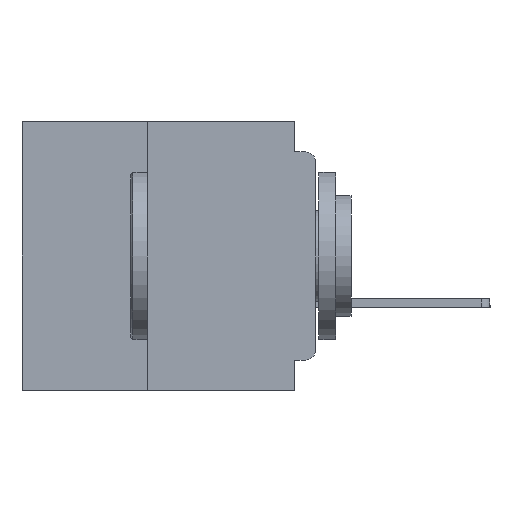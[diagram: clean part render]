
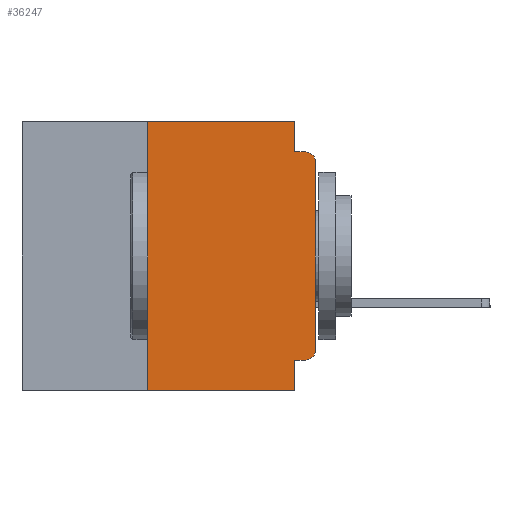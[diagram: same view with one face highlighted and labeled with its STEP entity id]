
A CAD part, left-side view. The second image highlights one B-rep face of the part: STEP entity #36247.
In plain terms, the highlighted planar face has unit normal (-1, 0, 0).
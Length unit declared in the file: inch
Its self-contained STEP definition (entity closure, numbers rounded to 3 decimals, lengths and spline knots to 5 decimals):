
#395 = ORIENTED_EDGE ( 'NONE', *, *, #25275, .F. ) ;
#446 = EDGE_CURVE ( 'NONE', #2039, #25079, #13232, .T. ) ;
#483 = VECTOR ( 'NONE', #23274, 39.37008 ) ;
#754 = AXIS2_PLACEMENT_3D ( 'NONE', #5023, #29631, #8598 ) ;
#2039 = VERTEX_POINT ( 'NONE', #27546 ) ;
#3503 = VECTOR ( 'NONE', #42438, 39.37008 ) ;
#3604 = CIRCLE ( 'NONE', #41711, 0.015 ) ;
#3723 = CARTESIAN_POINT ( 'NONE',  ( 0., 0., -0.06 ) ) ;
#4589 = LINE ( 'NONE', #10989, #3503 ) ;
#5023 = CARTESIAN_POINT ( 'NONE',  ( 0., 0.437, 0. ) ) ;
#5194 = CARTESIAN_POINT ( 'NONE',  ( 0., 0.031, -0.4 ) ) ;
#5878 = CARTESIAN_POINT ( 'NONE',  ( 0., 0.031, -0.4 ) ) ;
#6383 = CARTESIAN_POINT ( 'NONE',  ( 0., 0.031, -0.355 ) ) ;
#6879 = VECTOR ( 'NONE', #44340, 39.37008 ) ;
#7623 = LINE ( 'NONE', #41251, #25225 ) ;
#7993 = AXIS2_PLACEMENT_3D ( 'NONE', #16415, #40830, #19951 ) ;
#8598 = DIRECTION ( 'NONE',  ( 0., 0., -1. ) ) ;
#9558 = ORIENTED_EDGE ( 'NONE', *, *, #15839, .F. ) ;
#9812 = EDGE_LOOP ( 'NONE', ( #27201, #44619, #27132, #28868, #9558, #395, #15084, #21451, #10357, #39577 ) ) ;
#10357 = ORIENTED_EDGE ( 'NONE', *, *, #446, .F. ) ;
#10989 = CARTESIAN_POINT ( 'NONE',  ( 0., 0.25, -0.4 ) ) ;
#11476 = VERTEX_POINT ( 'NONE', #43487 ) ;
#11868 = VECTOR ( 'NONE', #21684, 39.37008 ) ;
#12279 = DIRECTION ( 'NONE',  ( 0., 0., 1. ) ) ;
#12887 = EDGE_CURVE ( 'NONE', #2039, #37448, #28032, .T. ) ;
#13232 = LINE ( 'NONE', #26518, #30829 ) ;
#13358 = VERTEX_POINT ( 'NONE', #26187 ) ;
#15084 = ORIENTED_EDGE ( 'NONE', *, *, #32418, .T. ) ;
#15514 = PLANE ( 'NONE',  #754 ) ;
#15839 = EDGE_CURVE ( 'NONE', #16154, #13358, #7623, .T. ) ;
#16154 = VERTEX_POINT ( 'NONE', #39728 ) ;
#16415 = CARTESIAN_POINT ( 'NONE',  ( 0., 0.015, -0.34 ) ) ;
#16901 = LINE ( 'NONE', #45179, #43590 ) ;
#17373 = DIRECTION ( 'NONE',  ( 0., -1., 0. ) ) ;
#17831 = DIRECTION ( 'NONE',  ( -1., 0., 0. ) ) ;
#18166 = EDGE_CURVE ( 'NONE', #13358, #20723, #30558, .T. ) ;
#18183 = CARTESIAN_POINT ( 'NONE',  ( 0., 0.031, 0. ) ) ;
#18848 = CARTESIAN_POINT ( 'NONE',  ( 0., 0.031, -0.045 ) ) ;
#19744 = CARTESIAN_POINT ( 'NONE',  ( 0., 0.437, -0.4 ) ) ;
#19951 = DIRECTION ( 'NONE',  ( 0., 0., -1. ) ) ;
#20604 = CARTESIAN_POINT ( 'NONE',  ( 0., 0.015, -0.045 ) ) ;
#20723 = VERTEX_POINT ( 'NONE', #18848 ) ;
#21451 = ORIENTED_EDGE ( 'NONE', *, *, #34818, .F. ) ;
#21684 = DIRECTION ( 'NONE',  ( 0., 0., -1. ) ) ;
#22727 = CARTESIAN_POINT ( 'NONE',  ( 0., 0., 0. ) ) ;
#23274 = DIRECTION ( 'NONE',  ( 0., -1., 0. ) ) ;
#24052 = DIRECTION ( 'NONE',  ( 0., -1., 0. ) ) ;
#25079 = VERTEX_POINT ( 'NONE', #6383 ) ;
#25225 = VECTOR ( 'NONE', #24052, 39.37008 ) ;
#25275 = EDGE_CURVE ( 'NONE', #11476, #16154, #4589, .T. ) ;
#26187 = CARTESIAN_POINT ( 'NONE',  ( 0., 0.031, 0. ) ) ;
#26315 = CARTESIAN_POINT ( 'NONE',  ( 0., 0., -0.34 ) ) ;
#26518 = CARTESIAN_POINT ( 'NONE',  ( 0., 0., -0.355 ) ) ;
#27132 = ORIENTED_EDGE ( 'NONE', *, *, #33754, .F. ) ;
#27201 = ORIENTED_EDGE ( 'NONE', *, *, #38030, .T. ) ;
#27368 = DIRECTION ( 'NONE',  ( 0., 1., 0. ) ) ;
#27546 = CARTESIAN_POINT ( 'NONE',  ( 0., 0.015, -0.355 ) ) ;
#28032 = CIRCLE ( 'NONE', #7993, 0.015 ) ;
#28575 = LINE ( 'NONE', #19744, #483 ) ;
#28802 = FACE_OUTER_BOUND ( 'NONE', #9812, .T. ) ;
#28868 = ORIENTED_EDGE ( 'NONE', *, *, #18166, .F. ) ;
#29631 = DIRECTION ( 'NONE',  ( 1., 0., 0. ) ) ;
#30558 = LINE ( 'NONE', #18183, #11868 ) ;
#30829 = VECTOR ( 'NONE', #27368, 39.37008 ) ;
#32418 = EDGE_CURVE ( 'NONE', #11476, #38021, #28575, .T. ) ;
#32707 = VERTEX_POINT ( 'NONE', #3723 ) ;
#33717 = VERTEX_POINT ( 'NONE', #20604 ) ;
#33754 = EDGE_CURVE ( 'NONE', #20723, #33717, #16901, .T. ) ;
#34818 = EDGE_CURVE ( 'NONE', #25079, #38021, #34927, .T. ) ;
#34927 = LINE ( 'NONE', #5878, #6879 ) ;
#36247 = ADVANCED_FACE ( 'NONE', ( #28802 ), #15514, .F. ) ;
#37250 = LINE ( 'NONE', #22727, #45234 ) ;
#37448 = VERTEX_POINT ( 'NONE', #26315 ) ;
#38021 = VERTEX_POINT ( 'NONE', #5194 ) ;
#38030 = EDGE_CURVE ( 'NONE', #37448, #32707, #37250, .T. ) ;
#38776 = CARTESIAN_POINT ( 'NONE',  ( 0., 0.015, -0.06 ) ) ;
#39440 = EDGE_CURVE ( 'NONE', #32707, #33717, #3604, .T. ) ;
#39577 = ORIENTED_EDGE ( 'NONE', *, *, #12887, .T. ) ;
#39728 = CARTESIAN_POINT ( 'NONE',  ( 0., 0.25, 0. ) ) ;
#40830 = DIRECTION ( 'NONE',  ( -1., 0., 0. ) ) ;
#41251 = CARTESIAN_POINT ( 'NONE',  ( 0., 0.437, 0. ) ) ;
#41711 = AXIS2_PLACEMENT_3D ( 'NONE', #38776, #17831, #42201 ) ;
#42201 = DIRECTION ( 'NONE',  ( 0., 0., -1. ) ) ;
#42438 = DIRECTION ( 'NONE',  ( 0., 0., 1. ) ) ;
#43487 = CARTESIAN_POINT ( 'NONE',  ( 0., 0.25, -0.4 ) ) ;
#43590 = VECTOR ( 'NONE', #17373, 39.37008 ) ;
#44340 = DIRECTION ( 'NONE',  ( 0., 0., -1. ) ) ;
#44619 = ORIENTED_EDGE ( 'NONE', *, *, #39440, .T. ) ;
#45179 = CARTESIAN_POINT ( 'NONE',  ( 0., 0., -0.045 ) ) ;
#45234 = VECTOR ( 'NONE', #12279, 39.37008 ) ;
